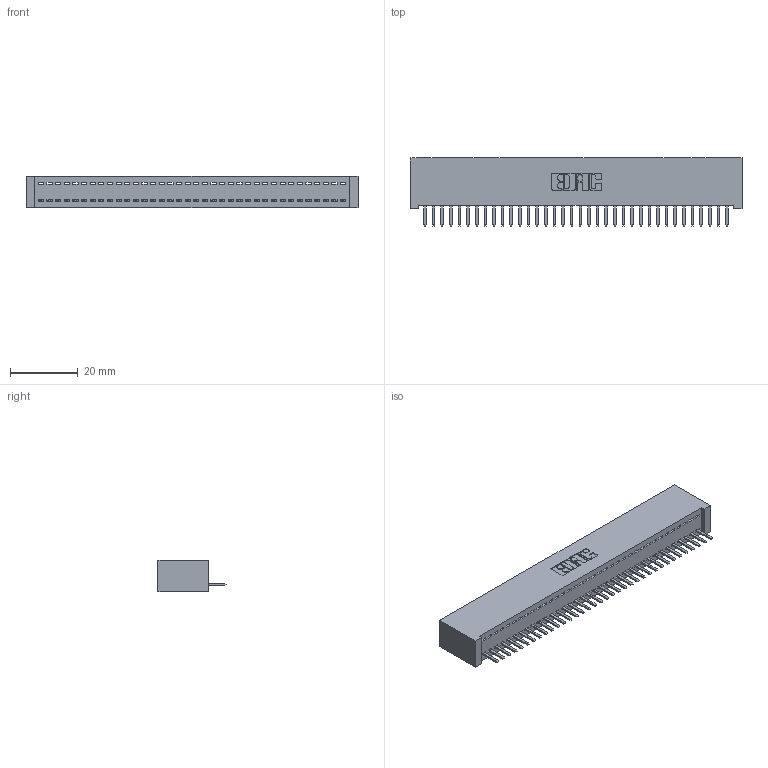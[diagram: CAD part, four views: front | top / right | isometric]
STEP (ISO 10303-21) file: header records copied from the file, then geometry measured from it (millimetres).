
FILE_DESCRIPTION (( 'STEP AP203' ), '1' );
FILE_NAME ('342-036-520-101.STEP', '2019-10-02T13:06:21', ( '' ), ( '' ), 'SwSTEP 2.0', 'SolidWorks 2016', '' );
FILE_SCHEMA (( 'CONFIG_CONTROL_DESIGN' ));
Length unit declared in the file: inch
Products named in the file (3): 342 Part_Lugless; 345-292-001_345-293-120; 342-036-520-101
Assembly tree (37 placements, depth 2):
  342-036-520-101
    342 Part_Lugless
    345-292-001_345-293-120  x36
Bounding box: 97.69 x 20.02 x 9.4 mm (x, y, z)
Volume: 8848.6 mm3; surface area: 12873.9 mm2
Topology: 37 solids, 37 shells, 2334 faces, 6899 edges, 4502 vertices
Faces by surface type: plane 1646, cylinder 688
Entity records: 22489 total; most frequent: CARTESIAN_POINT 3898, ORIENTED_EDGE 3858, DIRECTION 3281, EDGE_CURVE 1929, LINE 1805, VECTOR 1805, VERTEX_POINT 1282, AXIS2_PLACEMENT_3D 738
